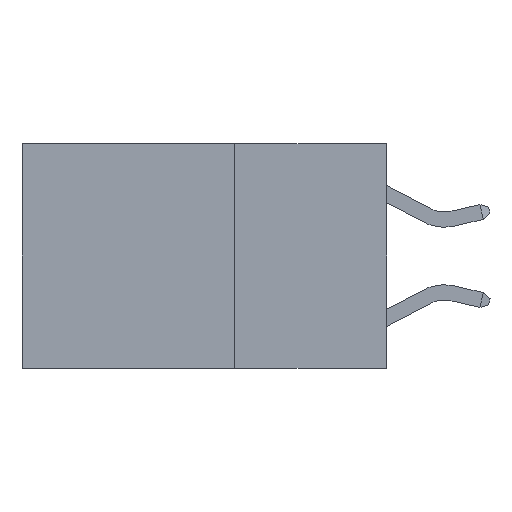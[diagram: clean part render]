
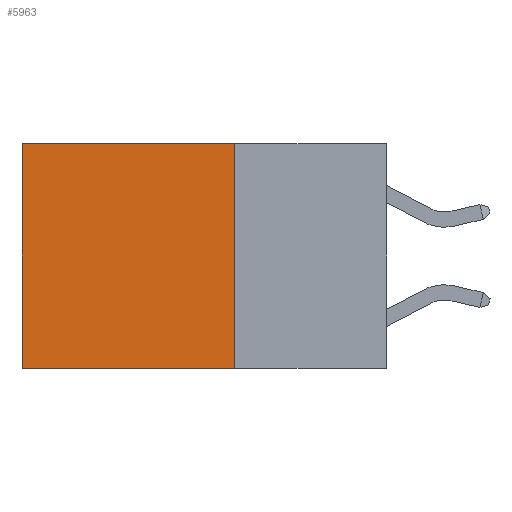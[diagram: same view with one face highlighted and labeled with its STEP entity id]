
A CAD part, left-side view. The second image highlights one B-rep face of the part: STEP entity #5963.
In plain terms, the highlighted planar face has unit normal (-1, 0, 0).
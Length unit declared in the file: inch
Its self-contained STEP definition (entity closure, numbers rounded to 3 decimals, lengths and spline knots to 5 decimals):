
#97 = DIRECTION ( 'NONE',  ( 0., 0., -1. ) ) ;
#440 = EDGE_CURVE ( 'NONE', #5285, #2068, #10912, .T. ) ;
#487 = CARTESIAN_POINT ( 'NONE',  ( 0.2625, 0.25, -0.37 ) ) ;
#1258 = LINE ( 'NONE', #8331, #3634 ) ;
#2068 = VERTEX_POINT ( 'NONE', #10307 ) ;
#2159 = VERTEX_POINT ( 'NONE', #6538 ) ;
#2452 = EDGE_CURVE ( 'NONE', #2159, #5285, #11602, .T. ) ;
#2633 = CARTESIAN_POINT ( 'NONE',  ( 0.2625, 0.6, 0. ) ) ;
#3383 = FACE_OUTER_BOUND ( 'NONE', #5577, .T. ) ;
#3493 = DIRECTION ( 'NONE',  ( 0., 1., 0. ) ) ;
#3564 = ORIENTED_EDGE ( 'NONE', *, *, #440, .F. ) ;
#3634 = VECTOR ( 'NONE', #3493, 39.37008 ) ;
#3989 = VECTOR ( 'NONE', #5491, 39.37008 ) ;
#4622 = CARTESIAN_POINT ( 'NONE',  ( 0.2625, 0.25, 0. ) ) ;
#5092 = CARTESIAN_POINT ( 'NONE',  ( 0.2625, 0.25, 0. ) ) ;
#5285 = VERTEX_POINT ( 'NONE', #487 ) ;
#5452 = VECTOR ( 'NONE', #9368, 39.37008 ) ;
#5491 = DIRECTION ( 'NONE',  ( 0., 0., -1. ) ) ;
#5577 = EDGE_LOOP ( 'NONE', ( #8319, #3564, #10568, #7495 ) ) ;
#5849 = VECTOR ( 'NONE', #10146, 39.37008 ) ;
#5963 = ADVANCED_FACE ( 'NONE', ( #3383 ), #11774, .F. ) ;
#6068 = DIRECTION ( 'NONE',  ( 1., 0., 0. ) ) ;
#6538 = CARTESIAN_POINT ( 'NONE',  ( 0.2625, 0.25, 0. ) ) ;
#7495 = ORIENTED_EDGE ( 'NONE', *, *, #10593, .T. ) ;
#8319 = ORIENTED_EDGE ( 'NONE', *, *, #9007, .T. ) ;
#8331 = CARTESIAN_POINT ( 'NONE',  ( 0.2625, 0.25, 0. ) ) ;
#8399 = VERTEX_POINT ( 'NONE', #11302 ) ;
#9007 = EDGE_CURVE ( 'NONE', #8399, #2068, #9943, .T. ) ;
#9368 = DIRECTION ( 'NONE',  ( 0., 0., -1. ) ) ;
#9943 = LINE ( 'NONE', #2633, #5452 ) ;
#10146 = DIRECTION ( 'NONE',  ( 0., 1., 0. ) ) ;
#10307 = CARTESIAN_POINT ( 'NONE',  ( 0.2625, 0.6, -0.37 ) ) ;
#10559 = CARTESIAN_POINT ( 'NONE',  ( 0.2625, 0.25, -0.37 ) ) ;
#10568 = ORIENTED_EDGE ( 'NONE', *, *, #2452, .F. ) ;
#10593 = EDGE_CURVE ( 'NONE', #2159, #8399, #1258, .T. ) ;
#10912 = LINE ( 'NONE', #10559, #5849 ) ;
#11302 = CARTESIAN_POINT ( 'NONE',  ( 0.2625, 0.6, 0. ) ) ;
#11602 = LINE ( 'NONE', #4622, #3989 ) ;
#11774 = PLANE ( 'NONE',  #11860 ) ;
#11860 = AXIS2_PLACEMENT_3D ( 'NONE', #5092, #6068, #97 ) ;
